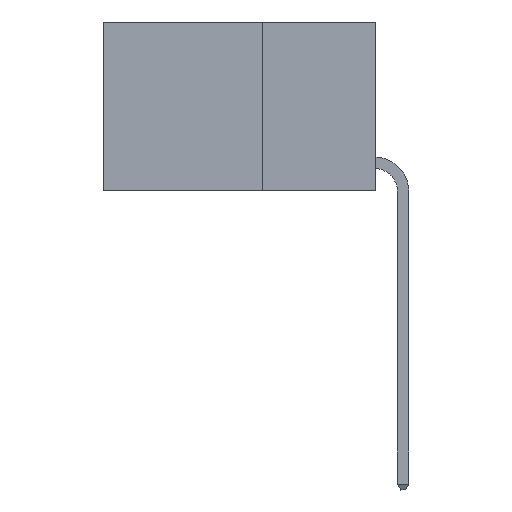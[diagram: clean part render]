
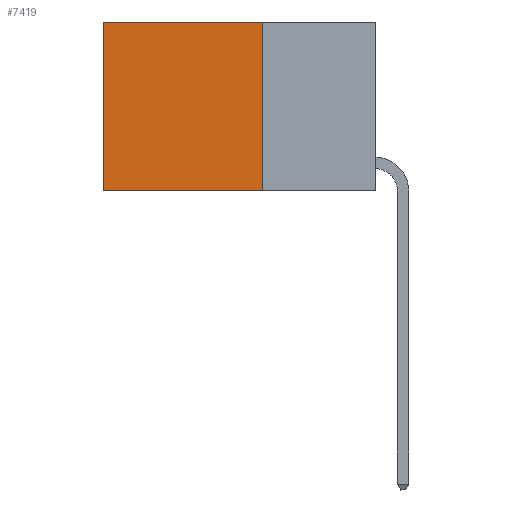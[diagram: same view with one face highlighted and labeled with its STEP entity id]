
A CAD part, left-side view. The second image highlights one B-rep face of the part: STEP entity #7419.
In plain terms, the highlighted planar face has unit normal (-1, 0, 0).
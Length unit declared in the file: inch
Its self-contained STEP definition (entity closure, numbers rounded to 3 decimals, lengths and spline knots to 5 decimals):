
#426 = VERTEX_POINT ( 'NONE', #12865 ) ;
#735 = LINE ( 'NONE', #10210, #2317 ) ;
#858 = CARTESIAN_POINT ( 'NONE',  ( 0.2625, 0.25, -0.37 ) ) ;
#1836 = CARTESIAN_POINT ( 'NONE',  ( 0.2625, 0.25, 0. ) ) ;
#2084 = VERTEX_POINT ( 'NONE', #9105 ) ;
#2317 = VECTOR ( 'NONE', #9051, 39.37008 ) ;
#2342 = CARTESIAN_POINT ( 'NONE',  ( 0.2625, 0.25, 0. ) ) ;
#3346 = VECTOR ( 'NONE', #6514, 39.37008 ) ;
#4228 = DIRECTION ( 'NONE',  ( 0., 1., 0. ) ) ;
#4312 = AXIS2_PLACEMENT_3D ( 'NONE', #1836, #11278, #10098 ) ;
#4624 = CARTESIAN_POINT ( 'NONE',  ( 0.2625, 0.25, -0.37 ) ) ;
#5352 = LINE ( 'NONE', #858, #12801 ) ;
#6132 = EDGE_LOOP ( 'NONE', ( #7417, #13182, #6644, #6191 ) ) ;
#6151 = VERTEX_POINT ( 'NONE', #4624 ) ;
#6191 = ORIENTED_EDGE ( 'NONE', *, *, #14460, .T. ) ;
#6455 = CARTESIAN_POINT ( 'NONE',  ( 0.2625, 0.6, 0. ) ) ;
#6514 = DIRECTION ( 'NONE',  ( 0., 0., -1. ) ) ;
#6644 = ORIENTED_EDGE ( 'NONE', *, *, #8264, .F. ) ;
#7417 = ORIENTED_EDGE ( 'NONE', *, *, #10956, .T. ) ;
#7419 = ADVANCED_FACE ( 'NONE', ( #8869 ), #7708, .F. ) ;
#7555 = CARTESIAN_POINT ( 'NONE',  ( 0.2625, 0.25, 0. ) ) ;
#7708 = PLANE ( 'NONE',  #4312 ) ;
#8264 = EDGE_CURVE ( 'NONE', #9838, #6151, #735, .T. ) ;
#8625 = LINE ( 'NONE', #7555, #8816 ) ;
#8772 = EDGE_CURVE ( 'NONE', #6151, #426, #5352, .T. ) ;
#8816 = VECTOR ( 'NONE', #4228, 39.37008 ) ;
#8869 = FACE_OUTER_BOUND ( 'NONE', #6132, .T. ) ;
#8906 = LINE ( 'NONE', #6455, #3346 ) ;
#9051 = DIRECTION ( 'NONE',  ( 0., 0., -1. ) ) ;
#9105 = CARTESIAN_POINT ( 'NONE',  ( 0.2625, 0.6, 0. ) ) ;
#9838 = VERTEX_POINT ( 'NONE', #2342 ) ;
#10098 = DIRECTION ( 'NONE',  ( 0., 0., -1. ) ) ;
#10210 = CARTESIAN_POINT ( 'NONE',  ( 0.2625, 0.25, 0. ) ) ;
#10956 = EDGE_CURVE ( 'NONE', #2084, #426, #8906, .T. ) ;
#11278 = DIRECTION ( 'NONE',  ( 1., 0., 0. ) ) ;
#12801 = VECTOR ( 'NONE', #14956, 39.37008 ) ;
#12865 = CARTESIAN_POINT ( 'NONE',  ( 0.2625, 0.6, -0.37 ) ) ;
#13182 = ORIENTED_EDGE ( 'NONE', *, *, #8772, .F. ) ;
#14460 = EDGE_CURVE ( 'NONE', #9838, #2084, #8625, .T. ) ;
#14956 = DIRECTION ( 'NONE',  ( 0., 1., 0. ) ) ;
